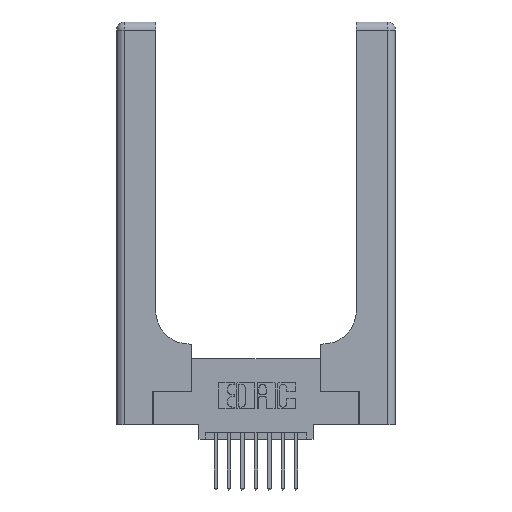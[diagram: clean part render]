
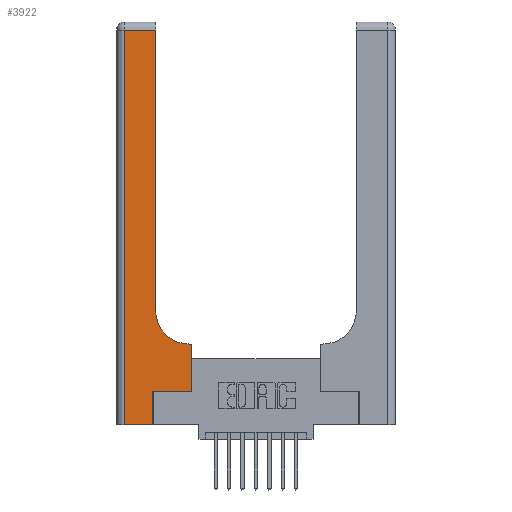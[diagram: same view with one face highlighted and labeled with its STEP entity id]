
A CAD part, top view. The second image highlights one B-rep face of the part: STEP entity #3922.
In plain terms, the highlighted planar face has unit normal (0, 0, 1).
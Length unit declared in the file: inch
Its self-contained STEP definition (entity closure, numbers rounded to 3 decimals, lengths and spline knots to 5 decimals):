
#240 = CARTESIAN_POINT ( 'NONE',  ( 0.2915, 3., 0.37 ) ) ;
#535 = VERTEX_POINT ( 'NONE', #14571 ) ;
#614 = CARTESIAN_POINT ( 'NONE',  ( 0.5585, 0.25, 0.37 ) ) ;
#1614 = LINE ( 'NONE', #1781, #7247 ) ;
#1656 = VECTOR ( 'NONE', #13367, 39.37008 ) ;
#1712 = VECTOR ( 'NONE', #11391, 39.37008 ) ;
#1781 = CARTESIAN_POINT ( 'NONE',  ( 0.06, 3., 0.37 ) ) ;
#1829 = DIRECTION ( 'NONE',  ( 0., -1., 0. ) ) ;
#2114 = VERTEX_POINT ( 'NONE', #15499 ) ;
#2148 = LINE ( 'NONE', #15123, #12457 ) ;
#2240 = ORIENTED_EDGE ( 'NONE', *, *, #2510, .T. ) ;
#2260 = LINE ( 'NONE', #13523, #11807 ) ;
#2305 = AXIS2_PLACEMENT_3D ( 'NONE', #10343, #6567, #7916 ) ;
#2510 = EDGE_CURVE ( 'NONE', #4029, #2114, #10859, .T. ) ;
#2913 = EDGE_CURVE ( 'NONE', #3925, #5971, #2260, .T. ) ;
#3004 = CARTESIAN_POINT ( 'NONE',  ( 0.2915, 0.6, 0.37 ) ) ;
#3007 = PLANE ( 'NONE',  #2305 ) ;
#3623 = EDGE_CURVE ( 'NONE', #12632, #9610, #4821, .T. ) ;
#3895 = VERTEX_POINT ( 'NONE', #11964 ) ;
#3922 = ADVANCED_FACE ( 'NONE', ( #9156 ), #3007, .F. ) ;
#3925 = VERTEX_POINT ( 'NONE', #614 ) ;
#3995 = ORIENTED_EDGE ( 'NONE', *, *, #10983, .T. ) ;
#4029 = VERTEX_POINT ( 'NONE', #7166 ) ;
#4382 = ORIENTED_EDGE ( 'NONE', *, *, #9901, .T. ) ;
#4387 = VECTOR ( 'NONE', #6398, 39.37008 ) ;
#4424 = EDGE_CURVE ( 'NONE', #535, #10218, #6902, .T. ) ;
#4752 = LINE ( 'NONE', #3004, #4387 ) ;
#4821 = LINE ( 'NONE', #10990, #1656 ) ;
#4945 = VECTOR ( 'NONE', #8549, 39.37008 ) ;
#5971 = VERTEX_POINT ( 'NONE', #11311 ) ;
#6132 = ORIENTED_EDGE ( 'NONE', *, *, #4424, .T. ) ;
#6297 = AXIS2_PLACEMENT_3D ( 'NONE', #12070, #14546, #13391 ) ;
#6398 = DIRECTION ( 'NONE',  ( -1., 0., 0. ) ) ;
#6567 = DIRECTION ( 'NONE',  ( 0., 0., -1. ) ) ;
#6902 = CIRCLE ( 'NONE', #6297, 0.25 ) ;
#7106 = CARTESIAN_POINT ( 'NONE',  ( 0.269, 0., 0.37 ) ) ;
#7166 = CARTESIAN_POINT ( 'NONE',  ( 0.06, 0., 0.37 ) ) ;
#7247 = VECTOR ( 'NONE', #1829, 39.37008 ) ;
#7834 = EDGE_LOOP ( 'NONE', ( #13976, #12838, #4382, #2240, #10415, #13377, #14166, #3995, #6132 ) ) ;
#7916 = DIRECTION ( 'NONE',  ( -1., 0., 0. ) ) ;
#8549 = DIRECTION ( 'NONE',  ( 0., 1., 0. ) ) ;
#8585 = CARTESIAN_POINT ( 'NONE',  ( 0.2915, 2.94, 0.37 ) ) ;
#9156 = FACE_OUTER_BOUND ( 'NONE', #7834, .T. ) ;
#9610 = VERTEX_POINT ( 'NONE', #14351 ) ;
#9901 = EDGE_CURVE ( 'NONE', #9610, #4029, #1614, .T. ) ;
#10048 = DIRECTION ( 'NONE',  ( 0., 1., 0. ) ) ;
#10218 = VERTEX_POINT ( 'NONE', #10762 ) ;
#10319 = EDGE_CURVE ( 'NONE', #10218, #12632, #11376, .T. ) ;
#10343 = CARTESIAN_POINT ( 'NONE',  ( 0., 3., 0.37 ) ) ;
#10415 = ORIENTED_EDGE ( 'NONE', *, *, #12696, .T. ) ;
#10762 = CARTESIAN_POINT ( 'NONE',  ( 0.2915, 0.85, 0.37 ) ) ;
#10859 = LINE ( 'NONE', #14983, #12164 ) ;
#10983 = EDGE_CURVE ( 'NONE', #5971, #535, #4752, .T. ) ;
#10990 = CARTESIAN_POINT ( 'NONE',  ( 0., 2.94, 0.37 ) ) ;
#11071 = EDGE_CURVE ( 'NONE', #3895, #3925, #2148, .T. ) ;
#11311 = CARTESIAN_POINT ( 'NONE',  ( 0.5585, 0.6, 0.37 ) ) ;
#11376 = LINE ( 'NONE', #240, #4945 ) ;
#11391 = DIRECTION ( 'NONE',  ( 0., 1., 0. ) ) ;
#11807 = VECTOR ( 'NONE', #10048, 39.37008 ) ;
#11964 = CARTESIAN_POINT ( 'NONE',  ( 0.269, 0.25, 0.37 ) ) ;
#12070 = CARTESIAN_POINT ( 'NONE',  ( 0.5415, 0.85, 0.37 ) ) ;
#12164 = VECTOR ( 'NONE', #14831, 39.37008 ) ;
#12457 = VECTOR ( 'NONE', #15166, 39.37008 ) ;
#12632 = VERTEX_POINT ( 'NONE', #8585 ) ;
#12696 = EDGE_CURVE ( 'NONE', #2114, #3895, #15240, .T. ) ;
#12838 = ORIENTED_EDGE ( 'NONE', *, *, #3623, .T. ) ;
#13367 = DIRECTION ( 'NONE',  ( -1., 0., 0. ) ) ;
#13377 = ORIENTED_EDGE ( 'NONE', *, *, #11071, .T. ) ;
#13391 = DIRECTION ( 'NONE',  ( 1., 0., 0. ) ) ;
#13523 = CARTESIAN_POINT ( 'NONE',  ( 0.5585, 0.25, 0.37 ) ) ;
#13976 = ORIENTED_EDGE ( 'NONE', *, *, #10319, .T. ) ;
#14166 = ORIENTED_EDGE ( 'NONE', *, *, #2913, .T. ) ;
#14351 = CARTESIAN_POINT ( 'NONE',  ( 0.06, 2.94, 0.37 ) ) ;
#14546 = DIRECTION ( 'NONE',  ( 0., 0., -1. ) ) ;
#14571 = CARTESIAN_POINT ( 'NONE',  ( 0.5415, 0.6, 0.37 ) ) ;
#14831 = DIRECTION ( 'NONE',  ( 1., 0., 0. ) ) ;
#14983 = CARTESIAN_POINT ( 'NONE',  ( 0., 0., 0.37 ) ) ;
#15123 = CARTESIAN_POINT ( 'NONE',  ( 0.269, 0.25, 0.37 ) ) ;
#15166 = DIRECTION ( 'NONE',  ( 1., 0., 0. ) ) ;
#15240 = LINE ( 'NONE', #7106, #1712 ) ;
#15499 = CARTESIAN_POINT ( 'NONE',  ( 0.269, 0., 0.37 ) ) ;
